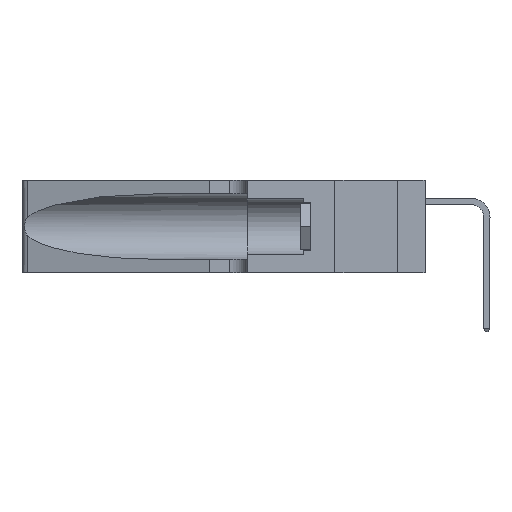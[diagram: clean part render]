
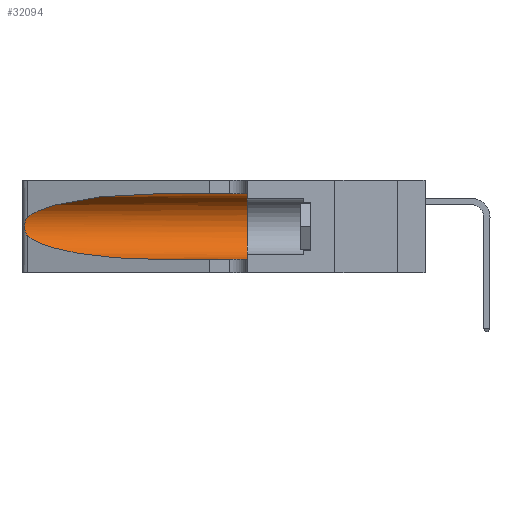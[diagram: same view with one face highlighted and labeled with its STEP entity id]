
A CAD part, left-side view. The second image highlights one B-rep face of the part: STEP entity #32094.
In plain terms, the highlighted cylindrical face has radius 3.308 mm (diameter 6.617 mm), a partial arc.
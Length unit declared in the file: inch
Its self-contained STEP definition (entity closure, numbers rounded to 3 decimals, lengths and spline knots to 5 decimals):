
#728 = CARTESIAN_POINT ( 'NONE',  ( 0.25789, 1.23486, 0.15765 ) ) ;
#1341 = ORIENTED_EDGE ( 'NONE', *, *, #30915, .F. ) ;
#1393 = VECTOR ( 'NONE', #17346, 39.37008 ) ;
#1762 = CARTESIAN_POINT ( 'NONE',  ( 0.1305, 0.72297, 0.31525 ) ) ;
#2861 = CARTESIAN_POINT ( 'NONE',  ( 0.2373, 1.15595, 0.08982 ) ) ;
#3364 = CARTESIAN_POINT ( 'NONE',  ( 0.25555, 1.22993, 0.14849 ) ) ;
#3541 = FACE_OUTER_BOUND ( 'NONE', #15294, .T. ) ;
#3592 = AXIS2_PLACEMENT_3D ( 'NONE', #30086, #12474, #22526 ) ;
#3905 = VERTEX_POINT ( 'NONE', #10484 ) ;
#4119 = CARTESIAN_POINT ( 'NONE',  ( 0.1305, 0.35, 0.31525 ) ) ;
#4388 = VERTEX_POINT ( 'NONE', #12195 ) ;
#4728 = CARTESIAN_POINT ( 'NONE',  ( 0.1305, 1.61858, 0.31525 ) ) ;
#5466 = ORIENTED_EDGE ( 'NONE', *, *, #27467, .F. ) ;
#5476 = CARTESIAN_POINT ( 'NONE',  ( 0.18966, 0.96281, 0.05475 ) ) ;
#5779 = VECTOR ( 'NONE', #8490, 39.37008 ) ;
#7993 = CIRCLE ( 'NONE', #17996, 0.13025 ) ;
#8350 = CARTESIAN_POINT ( 'NONE',  ( 0.25787, 1.23484, 0.2124 ) ) ;
#8490 = DIRECTION ( 'NONE',  ( 0., -1., 0. ) ) ;
#9700 = CARTESIAN_POINT ( 'NONE',  ( 0.2373, 1.15595, 0.28018 ) ) ;
#9730 = ORIENTED_EDGE ( 'NONE', *, *, #11978, .T. ) ;
#10484 = CARTESIAN_POINT ( 'NONE',  ( 0.1305, 0.35, 0.05475 ) ) ;
#10573 = CARTESIAN_POINT ( 'NONE',  ( 0.1305, 0.35, 0.185 ) ) ;
#10888 = CARTESIAN_POINT ( 'NONE',  ( 0.26018, 1.23835, 0.19895 ) ) ;
#11965 = VERTEX_POINT ( 'NONE', #20984 ) ;
#11978 = EDGE_CURVE ( 'NONE', #11965, #3905, #31726, .T. ) ;
#12195 = CARTESIAN_POINT ( 'NONE',  ( 0.1305, 0.72297, 0.31525 ) ) ;
#12474 = DIRECTION ( 'NONE',  ( 0., -1., 0. ) ) ;
#13103 = DIRECTION ( 'NONE',  ( 0., 0., 1. ) ) ;
#13414 = CARTESIAN_POINT ( 'NONE',  ( 0.26075, 1.23896, 0.178 ) ) ;
#15294 = EDGE_LOOP ( 'NONE', ( #27003, #17614, #25104, #9730, #1341, #5466 ) ) ;
#15467 = EDGE_CURVE ( 'NONE', #19701, #11965, #18327, .T. ) ;
#15731 = LINE ( 'NONE', #4728, #1393 ) ;
#15965 = CARTESIAN_POINT ( 'NONE',  ( 0.25856, 1.23593, 0.16098 ) ) ;
#17346 = DIRECTION ( 'NONE',  ( 0., -1., 0. ) ) ;
#17614 = ORIENTED_EDGE ( 'NONE', *, *, #22777, .T. ) ;
#17996 = AXIS2_PLACEMENT_3D ( 'NONE', #10573, #28169, #13103 ) ;
#18327 =( BOUNDED_CURVE ( )  B_SPLINE_CURVE ( 3, ( #20603, #2861, #5476, #23109 ),
 .UNSPECIFIED., .F., .F. ) 
 B_SPLINE_CURVE_WITH_KNOTS ( ( 4, 4 ),
 ( 3.44316, 4.71239 ),
 .UNSPECIFIED. ) 
 CURVE ( )  GEOMETRIC_REPRESENTATION_ITEM ( )  RATIONAL_B_SPLINE_CURVE ( ( 1., 0.87, 0.87, 1. ) ) 
 REPRESENTATION_ITEM ( '' )  );
#18527 = CARTESIAN_POINT ( 'NONE',  ( 0.25639, 1.23186, 0.15144 ) ) ;
#19701 = VERTEX_POINT ( 'NONE', #27395 ) ;
#19772 = CARTESIAN_POINT ( 'NONE',  ( 0.18966, 0.96281, 0.31525 ) ) ;
#20189 = VERTEX_POINT ( 'NONE', #4119 ) ;
#20603 = CARTESIAN_POINT ( 'NONE',  ( 0.25487, 1.22718, 0.14631 ) ) ;
#20942 = CARTESIAN_POINT ( 'NONE',  ( 0.25555, 1.22994, 0.2215 ) ) ;
#20984 = CARTESIAN_POINT ( 'NONE',  ( 0.1305, 0.72297, 0.05475 ) ) ;
#21047 = CARTESIAN_POINT ( 'NONE',  ( 0.25487, 1.22718, 0.14631 ) ) ;
#21738 = B_SPLINE_CURVE_WITH_KNOTS ( 'NONE', 3,
 ( #25861, #20942, #23446, #8350, #25965, #10888, #28494, #13414, #30998, #15965, #728, #18527, #3364, #21047 ),
 .UNSPECIFIED., .F., .F.,
 ( 4, 2, 2, 2, 2, 2, 4 ),
 ( 0., 0.00027, 0.00053, 0.00107, 0.0016, 0.00187, 0.00214 ),
 .UNSPECIFIED. ) ;
#22526 = DIRECTION ( 'NONE',  ( 0., 0., -1. ) ) ;
#22777 = EDGE_CURVE ( 'NONE', #32509, #19701, #21738, .T. ) ;
#23109 = CARTESIAN_POINT ( 'NONE',  ( 0.1305, 0.72297, 0.05475 ) ) ;
#23446 = CARTESIAN_POINT ( 'NONE',  ( 0.25639, 1.23184, 0.21858 ) ) ;
#23589 = CARTESIAN_POINT ( 'NONE',  ( 0.1305, 1.61858, 0.05475 ) ) ;
#24137 = CARTESIAN_POINT ( 'NONE',  ( 0.25487, 1.22718, 0.22369 ) ) ;
#24968 =( BOUNDED_CURVE ( )  B_SPLINE_CURVE ( 3, ( #1762, #19772, #9700, #27308 ),
 .UNSPECIFIED., .F., .T. ) 
 B_SPLINE_CURVE_WITH_KNOTS ( ( 4, 4 ),
 ( 1.5708, 2.84003 ),
 .UNSPECIFIED. ) 
 CURVE ( )  GEOMETRIC_REPRESENTATION_ITEM ( )  RATIONAL_B_SPLINE_CURVE ( ( 1., 0.87, 0.87, 1. ) ) 
 REPRESENTATION_ITEM ( '' )  );
#25104 = ORIENTED_EDGE ( 'NONE', *, *, #15467, .T. ) ;
#25861 = CARTESIAN_POINT ( 'NONE',  ( 0.25487, 1.22718, 0.22369 ) ) ;
#25965 = CARTESIAN_POINT ( 'NONE',  ( 0.25854, 1.2359, 0.20912 ) ) ;
#27003 = ORIENTED_EDGE ( 'NONE', *, *, #27431, .T. ) ;
#27308 = CARTESIAN_POINT ( 'NONE',  ( 0.25487, 1.22718, 0.22369 ) ) ;
#27395 = CARTESIAN_POINT ( 'NONE',  ( 0.25487, 1.22718, 0.14631 ) ) ;
#27431 = EDGE_CURVE ( 'NONE', #4388, #32509, #24968, .T. ) ;
#27467 = EDGE_CURVE ( 'NONE', #4388, #20189, #15731, .T. ) ;
#28169 = DIRECTION ( 'NONE',  ( 0., 1., 0. ) ) ;
#28494 = CARTESIAN_POINT ( 'NONE',  ( 0.26075, 1.23896, 0.19203 ) ) ;
#30086 = CARTESIAN_POINT ( 'NONE',  ( 0.1305, 1.61858, 0.185 ) ) ;
#30915 = EDGE_CURVE ( 'NONE', #20189, #3905, #7993, .T. ) ;
#30998 = CARTESIAN_POINT ( 'NONE',  ( 0.26017, 1.23833, 0.17102 ) ) ;
#31726 = LINE ( 'NONE', #23589, #5779 ) ;
#32094 = ADVANCED_FACE ( 'NONE', ( #3541 ), #32127, .F. ) ;
#32127 = CYLINDRICAL_SURFACE ( 'NONE', #3592, 0.13025 ) ;
#32509 = VERTEX_POINT ( 'NONE', #24137 ) ;
